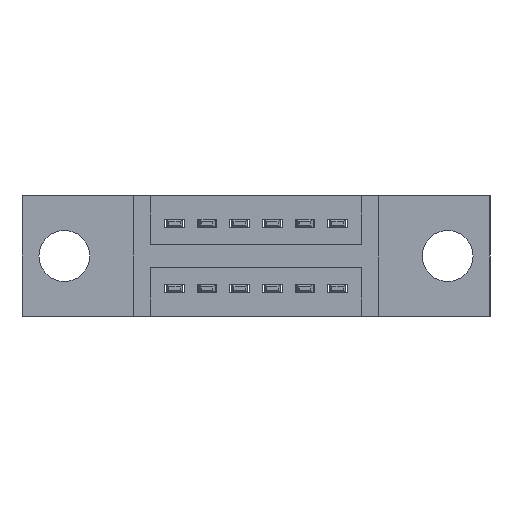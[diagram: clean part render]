
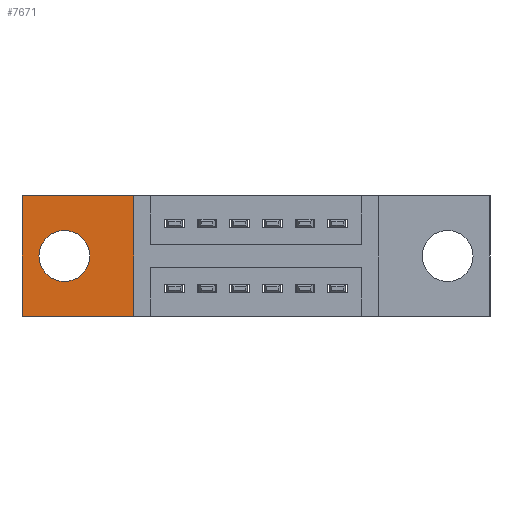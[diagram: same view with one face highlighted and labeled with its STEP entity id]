
A CAD part, front view. The second image highlights one B-rep face of the part: STEP entity #7671.
In plain terms, the highlighted planar face has unit normal (0, -1, 0).
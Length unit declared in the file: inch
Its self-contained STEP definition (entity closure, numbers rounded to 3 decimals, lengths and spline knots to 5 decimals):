
#371 = ORIENTED_EDGE ( 'NONE', *, *, #983, .F. ) ;
#534 = EDGE_LOOP ( 'NONE', ( #371, #7562 ) ) ;
#759 = CIRCLE ( 'NONE', #6361, 0.078 ) ;
#871 = DIRECTION ( 'NONE',  ( 0., 0., -1. ) ) ;
#983 = EDGE_CURVE ( 'NONE', #8942, #3433, #6496, .T. ) ;
#1009 = DIRECTION ( 'NONE',  ( 0., -1., 0. ) ) ;
#1031 = EDGE_CURVE ( 'NONE', #3433, #8942, #759, .T. ) ;
#1402 = VECTOR ( 'NONE', #6749, 39.37008 ) ;
#1426 = EDGE_CURVE ( 'NONE', #4583, #9341, #5723, .T. ) ;
#1516 = LINE ( 'NONE', #7577, #6840 ) ;
#1628 = PLANE ( 'NONE',  #9756 ) ;
#2014 = VECTOR ( 'NONE', #7962, 39.37008 ) ;
#2258 = ORIENTED_EDGE ( 'NONE', *, *, #6615, .T. ) ;
#2338 = CARTESIAN_POINT ( 'NONE',  ( 0.13, 0.11, -0.107 ) ) ;
#2425 = DIRECTION ( 'NONE',  ( 0., -1., 0. ) ) ;
#2499 = LINE ( 'NONE', #6354, #2014 ) ;
#2552 = VERTEX_POINT ( 'NONE', #3843 ) ;
#2555 = CARTESIAN_POINT ( 'NONE',  ( 0., 0.11, -0.37 ) ) ;
#2802 = ORIENTED_EDGE ( 'NONE', *, *, #5781, .T. ) ;
#3105 = EDGE_CURVE ( 'NONE', #6278, #2552, #2499, .T. ) ;
#3433 = VERTEX_POINT ( 'NONE', #5281 ) ;
#3634 = DIRECTION ( 'NONE',  ( 0., 0., -1. ) ) ;
#3714 = LINE ( 'NONE', #9171, #1402 ) ;
#3843 = CARTESIAN_POINT ( 'NONE',  ( 0., 0.11, 0. ) ) ;
#4107 = AXIS2_PLACEMENT_3D ( 'NONE', #6462, #1009, #7110 ) ;
#4439 = ORIENTED_EDGE ( 'NONE', *, *, #1426, .T. ) ;
#4489 = DIRECTION ( 'NONE',  ( 0., -1., 0. ) ) ;
#4583 = VERTEX_POINT ( 'NONE', #8219 ) ;
#5186 = ORIENTED_EDGE ( 'NONE', *, *, #3105, .T. ) ;
#5281 = CARTESIAN_POINT ( 'NONE',  ( 0.13, 0.11, -0.263 ) ) ;
#5402 = CARTESIAN_POINT ( 'NONE',  ( 0.3425, 0.11, 0. ) ) ;
#5585 = DIRECTION ( 'NONE',  ( 1., 0., 0. ) ) ;
#5723 = LINE ( 'NONE', #2555, #8185 ) ;
#5781 = EDGE_CURVE ( 'NONE', #2552, #4583, #3714, .T. ) ;
#6162 = EDGE_LOOP ( 'NONE', ( #2802, #4439, #2258, #5186 ) ) ;
#6278 = VERTEX_POINT ( 'NONE', #5402 ) ;
#6354 = CARTESIAN_POINT ( 'NONE',  ( 0., 0.11, 0. ) ) ;
#6361 = AXIS2_PLACEMENT_3D ( 'NONE', #8293, #4489, #3634 ) ;
#6462 = CARTESIAN_POINT ( 'NONE',  ( 0.13, 0.11, -0.185 ) ) ;
#6496 = CIRCLE ( 'NONE', #4107, 0.078 ) ;
#6615 = EDGE_CURVE ( 'NONE', #9341, #6278, #1516, .T. ) ;
#6749 = DIRECTION ( 'NONE',  ( 0., 0., -1. ) ) ;
#6840 = VECTOR ( 'NONE', #9843, 39.37008 ) ;
#7110 = DIRECTION ( 'NONE',  ( 0., 0., -1. ) ) ;
#7562 = ORIENTED_EDGE ( 'NONE', *, *, #1031, .F. ) ;
#7577 = CARTESIAN_POINT ( 'NONE',  ( 0.3425, 0.11, 0. ) ) ;
#7671 = ADVANCED_FACE ( 'NONE', ( #8506, #9307 ), #1628, .T. ) ;
#7747 = CARTESIAN_POINT ( 'NONE',  ( 0., 0.11, -0.37 ) ) ;
#7962 = DIRECTION ( 'NONE',  ( -1., 0., 0. ) ) ;
#8185 = VECTOR ( 'NONE', #5585, 39.37008 ) ;
#8219 = CARTESIAN_POINT ( 'NONE',  ( 0., 0.11, -0.37 ) ) ;
#8293 = CARTESIAN_POINT ( 'NONE',  ( 0.13, 0.11, -0.185 ) ) ;
#8506 = FACE_BOUND ( 'NONE', #534, .T. ) ;
#8734 = CARTESIAN_POINT ( 'NONE',  ( 0.3425, 0.11, -0.37 ) ) ;
#8942 = VERTEX_POINT ( 'NONE', #2338 ) ;
#9171 = CARTESIAN_POINT ( 'NONE',  ( 0., 0.11, 0. ) ) ;
#9307 = FACE_OUTER_BOUND ( 'NONE', #6162, .T. ) ;
#9341 = VERTEX_POINT ( 'NONE', #8734 ) ;
#9756 = AXIS2_PLACEMENT_3D ( 'NONE', #7747, #2425, #871 ) ;
#9843 = DIRECTION ( 'NONE',  ( 0., 0., 1. ) ) ;
